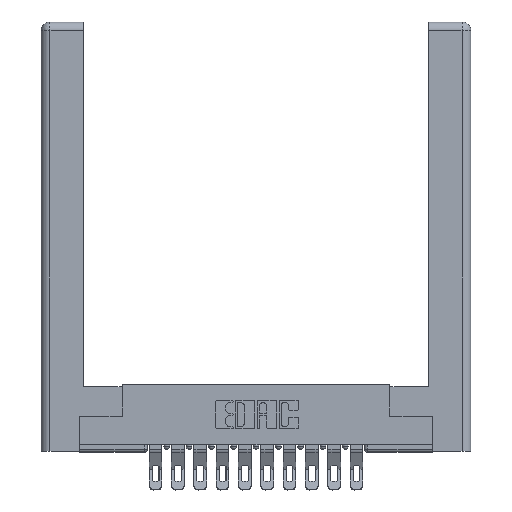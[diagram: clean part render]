
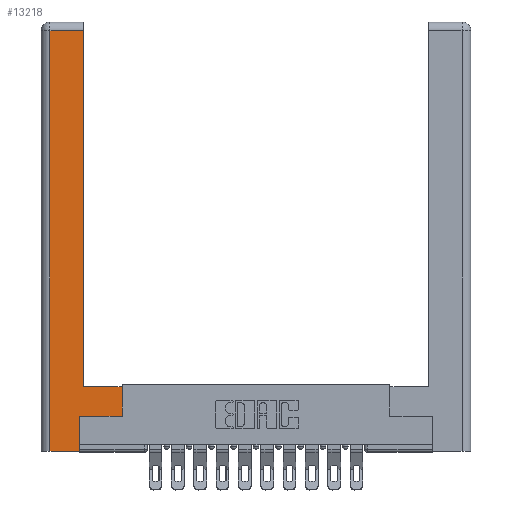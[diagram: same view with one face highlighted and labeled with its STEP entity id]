
A CAD part, top view. The second image highlights one B-rep face of the part: STEP entity #13218.
In plain terms, the highlighted planar face has unit normal (0, 0, 1).
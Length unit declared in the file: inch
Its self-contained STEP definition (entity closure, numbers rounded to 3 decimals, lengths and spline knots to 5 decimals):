
#846 = DIRECTION ( 'NONE',  ( -1., 0., 0. ) ) ;
#1104 = LINE ( 'NONE', #2561, #11537 ) ;
#1155 = VERTEX_POINT ( 'NONE', #15259 ) ;
#1163 = ORIENTED_EDGE ( 'NONE', *, *, #6044, .T. ) ;
#1552 = CARTESIAN_POINT ( 'NONE',  ( 0.295, 0.45, 0. ) ) ;
#2122 = DIRECTION ( 'NONE',  ( -1., 0., 0. ) ) ;
#2268 = ORIENTED_EDGE ( 'NONE', *, *, #10033, .T. ) ;
#2467 = DIRECTION ( 'NONE',  ( 0., 0., -1. ) ) ;
#2480 = ORIENTED_EDGE ( 'NONE', *, *, #15962, .T. ) ;
#2492 = CARTESIAN_POINT ( 'NONE',  ( 0.565, 0.245, 0. ) ) ;
#2561 = CARTESIAN_POINT ( 'NONE',  ( 0.265, 0.245, 0. ) ) ;
#2620 = VECTOR ( 'NONE', #11786, 39.37008 ) ;
#2843 = VERTEX_POINT ( 'NONE', #8780 ) ;
#4149 = VECTOR ( 'NONE', #9441, 39.37008 ) ;
#4162 = CARTESIAN_POINT ( 'NONE',  ( 0.565, 0.45, 0. ) ) ;
#4669 = CARTESIAN_POINT ( 'NONE',  ( 0.295, 3., 0. ) ) ;
#5369 = ORIENTED_EDGE ( 'NONE', *, *, #11672, .T. ) ;
#5732 = VERTEX_POINT ( 'NONE', #10254 ) ;
#5807 = CARTESIAN_POINT ( 'NONE',  ( 0.265, 0., 0. ) ) ;
#5914 = LINE ( 'NONE', #11030, #13361 ) ;
#6044 = EDGE_CURVE ( 'NONE', #15181, #2843, #7422, .T. ) ;
#6196 = CARTESIAN_POINT ( 'NONE',  ( 0., 0., 0. ) ) ;
#6219 = EDGE_CURVE ( 'NONE', #5732, #8592, #11231, .T. ) ;
#6681 = AXIS2_PLACEMENT_3D ( 'NONE', #6196, #2467, #7415 ) ;
#6693 = VERTEX_POINT ( 'NONE', #1552 ) ;
#7021 = LINE ( 'NONE', #10504, #12445 ) ;
#7260 = EDGE_CURVE ( 'NONE', #6693, #1155, #15761, .T. ) ;
#7261 = CARTESIAN_POINT ( 'NONE',  ( 0.0615, 0., 0. ) ) ;
#7326 = EDGE_CURVE ( 'NONE', #8592, #6693, #7021, .T. ) ;
#7415 = DIRECTION ( 'NONE',  ( -1., 0., 0. ) ) ;
#7422 = LINE ( 'NONE', #7261, #7866 ) ;
#7426 = ORIENTED_EDGE ( 'NONE', *, *, #7260, .T. ) ;
#7866 = VECTOR ( 'NONE', #14611, 39.37008 ) ;
#8376 = VECTOR ( 'NONE', #9017, 39.37008 ) ;
#8592 = VERTEX_POINT ( 'NONE', #11490 ) ;
#8780 = CARTESIAN_POINT ( 'NONE',  ( 0.0615, 0., 0. ) ) ;
#9017 = DIRECTION ( 'NONE',  ( 0., 1., 0. ) ) ;
#9396 = CARTESIAN_POINT ( 'NONE',  ( 0.0615, 2.94, 0. ) ) ;
#9441 = DIRECTION ( 'NONE',  ( 0., 1., 0. ) ) ;
#9464 = ORIENTED_EDGE ( 'NONE', *, *, #12577, .T. ) ;
#9686 = CARTESIAN_POINT ( 'NONE',  ( 0.265, 0.245, 0. ) ) ;
#10033 = EDGE_CURVE ( 'NONE', #10404, #5732, #13499, .T. ) ;
#10254 = CARTESIAN_POINT ( 'NONE',  ( 0.565, 0.245, 0. ) ) ;
#10404 = VERTEX_POINT ( 'NONE', #9686 ) ;
#10504 = CARTESIAN_POINT ( 'NONE',  ( 0.295, 0.45, 0. ) ) ;
#11030 = CARTESIAN_POINT ( 'NONE',  ( 0.0615, 2.94, 0. ) ) ;
#11220 = VERTEX_POINT ( 'NONE', #5807 ) ;
#11231 = LINE ( 'NONE', #4162, #8376 ) ;
#11490 = CARTESIAN_POINT ( 'NONE',  ( 0.565, 0.45, 0. ) ) ;
#11537 = VECTOR ( 'NONE', #13642, 39.37008 ) ;
#11672 = EDGE_CURVE ( 'NONE', #11220, #10404, #1104, .T. ) ;
#11706 = ORIENTED_EDGE ( 'NONE', *, *, #6219, .T. ) ;
#11786 = DIRECTION ( 'NONE',  ( 1., 0., 0. ) ) ;
#12445 = VECTOR ( 'NONE', #846, 39.37008 ) ;
#12576 = EDGE_LOOP ( 'NONE', ( #7426, #9464, #1163, #2480, #5369, #2268, #11706, #13151 ) ) ;
#12577 = EDGE_CURVE ( 'NONE', #1155, #15181, #5914, .T. ) ;
#12827 = CARTESIAN_POINT ( 'NONE',  ( 0.265, 0., 0. ) ) ;
#12988 = LINE ( 'NONE', #12827, #2620 ) ;
#13151 = ORIENTED_EDGE ( 'NONE', *, *, #7326, .T. ) ;
#13218 = ADVANCED_FACE ( 'NONE', ( #14526 ), #13560, .F. ) ;
#13361 = VECTOR ( 'NONE', #2122, 39.37008 ) ;
#13499 = LINE ( 'NONE', #2492, #13613 ) ;
#13560 = PLANE ( 'NONE',  #6681 ) ;
#13613 = VECTOR ( 'NONE', #15856, 39.37008 ) ;
#13642 = DIRECTION ( 'NONE',  ( 0., 1., 0. ) ) ;
#14526 = FACE_OUTER_BOUND ( 'NONE', #12576, .T. ) ;
#14611 = DIRECTION ( 'NONE',  ( 0., -1., 0. ) ) ;
#15181 = VERTEX_POINT ( 'NONE', #9396 ) ;
#15259 = CARTESIAN_POINT ( 'NONE',  ( 0.295, 2.94, 0. ) ) ;
#15761 = LINE ( 'NONE', #4669, #4149 ) ;
#15856 = DIRECTION ( 'NONE',  ( 1., 0., 0. ) ) ;
#15962 = EDGE_CURVE ( 'NONE', #2843, #11220, #12988, .T. ) ;
